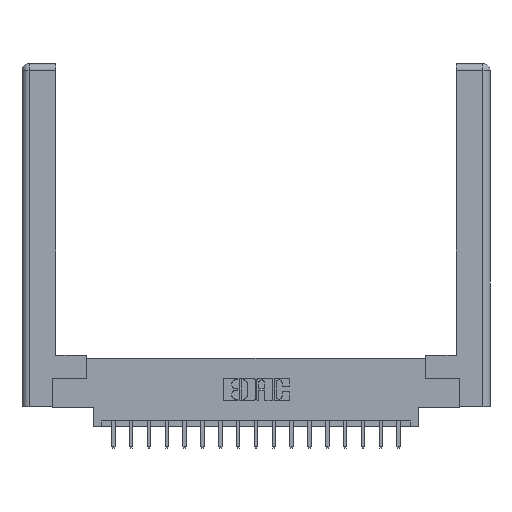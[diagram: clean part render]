
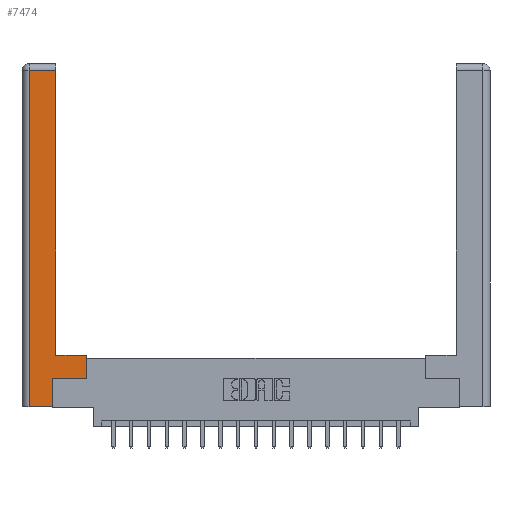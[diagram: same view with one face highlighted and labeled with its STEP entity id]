
A CAD part, top view. The second image highlights one B-rep face of the part: STEP entity #7474.
In plain terms, the highlighted planar face has unit normal (0, 0, 1).
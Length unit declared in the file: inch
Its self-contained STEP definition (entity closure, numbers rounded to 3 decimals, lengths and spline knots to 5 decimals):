
#240 = CARTESIAN_POINT ( 'NONE',  ( 0.295, 3., 0. ) ) ;
#743 = CARTESIAN_POINT ( 'NONE',  ( 0.295, 0.45, 0. ) ) ;
#848 = ORIENTED_EDGE ( 'NONE', *, *, #8095, .T. ) ;
#1612 = EDGE_LOOP ( 'NONE', ( #6051, #14851, #3664, #1820, #11303, #848, #16238, #18744 ) ) ;
#1820 = ORIENTED_EDGE ( 'NONE', *, *, #12712, .T. ) ;
#1840 = CARTESIAN_POINT ( 'NONE',  ( 0.565, 0.45, 0. ) ) ;
#2045 = EDGE_CURVE ( 'NONE', #13140, #7228, #2820, .T. ) ;
#2797 = VECTOR ( 'NONE', #11069, 39.37008 ) ;
#2820 = LINE ( 'NONE', #240, #8913 ) ;
#3087 = VERTEX_POINT ( 'NONE', #5712 ) ;
#3099 = AXIS2_PLACEMENT_3D ( 'NONE', #17085, #12384, #15464 ) ;
#3273 = LINE ( 'NONE', #4502, #3928 ) ;
#3664 = ORIENTED_EDGE ( 'NONE', *, *, #7607, .T. ) ;
#3837 = PLANE ( 'NONE',  #3099 ) ;
#3928 = VECTOR ( 'NONE', #10180, 39.37008 ) ;
#4420 = FACE_OUTER_BOUND ( 'NONE', #1612, .T. ) ;
#4452 = CARTESIAN_POINT ( 'NONE',  ( 0.0615, 2.94, 0. ) ) ;
#4502 = CARTESIAN_POINT ( 'NONE',  ( 0.265, 0.245, 0. ) ) ;
#4542 = CARTESIAN_POINT ( 'NONE',  ( 0.565, 0.245, 0. ) ) ;
#5068 = CARTESIAN_POINT ( 'NONE',  ( 0.295, 0.45, 0. ) ) ;
#5265 = VECTOR ( 'NONE', #14887, 39.37008 ) ;
#5712 = CARTESIAN_POINT ( 'NONE',  ( 0.265, 0., 0. ) ) ;
#6051 = ORIENTED_EDGE ( 'NONE', *, *, #2045, .T. ) ;
#6334 = DIRECTION ( 'NONE',  ( 0., 1., 0. ) ) ;
#6375 = LINE ( 'NONE', #1840, #14058 ) ;
#7228 = VERTEX_POINT ( 'NONE', #14047 ) ;
#7271 = VERTEX_POINT ( 'NONE', #15995 ) ;
#7474 = ADVANCED_FACE ( 'NONE', ( #4420 ), #3837, .F. ) ;
#7607 = EDGE_CURVE ( 'NONE', #18257, #17679, #17495, .T. ) ;
#7945 = DIRECTION ( 'NONE',  ( 0., 1., 0. ) ) ;
#8095 = EDGE_CURVE ( 'NONE', #7271, #8157, #14206, .T. ) ;
#8157 = VERTEX_POINT ( 'NONE', #4542 ) ;
#8913 = VECTOR ( 'NONE', #6334, 39.37008 ) ;
#9352 = LINE ( 'NONE', #743, #2797 ) ;
#9545 = DIRECTION ( 'NONE',  ( 0., -1., 0. ) ) ;
#9573 = VECTOR ( 'NONE', #9545, 39.37008 ) ;
#9794 = EDGE_CURVE ( 'NONE', #17604, #13140, #9352, .T. ) ;
#10180 = DIRECTION ( 'NONE',  ( 0., 1., 0. ) ) ;
#10429 = EDGE_CURVE ( 'NONE', #3087, #7271, #3273, .T. ) ;
#11069 = DIRECTION ( 'NONE',  ( -1., 0., 0. ) ) ;
#11303 = ORIENTED_EDGE ( 'NONE', *, *, #10429, .T. ) ;
#11360 = CARTESIAN_POINT ( 'NONE',  ( 0.565, 0.45, 0. ) ) ;
#11549 = LINE ( 'NONE', #4452, #5265 ) ;
#12154 = EDGE_CURVE ( 'NONE', #7228, #18257, #11549, .T. ) ;
#12261 = VECTOR ( 'NONE', #18531, 39.37008 ) ;
#12326 = VECTOR ( 'NONE', #19212, 39.37008 ) ;
#12384 = DIRECTION ( 'NONE',  ( 0., 0., -1. ) ) ;
#12712 = EDGE_CURVE ( 'NONE', #17679, #3087, #17409, .T. ) ;
#13140 = VERTEX_POINT ( 'NONE', #5068 ) ;
#14047 = CARTESIAN_POINT ( 'NONE',  ( 0.295, 2.94, 0. ) ) ;
#14058 = VECTOR ( 'NONE', #7945, 39.37008 ) ;
#14081 = CARTESIAN_POINT ( 'NONE',  ( 0.265, 0., 0. ) ) ;
#14206 = LINE ( 'NONE', #14645, #12326 ) ;
#14210 = CARTESIAN_POINT ( 'NONE',  ( 0.0615, 0., 0. ) ) ;
#14645 = CARTESIAN_POINT ( 'NONE',  ( 0.565, 0.245, 0. ) ) ;
#14851 = ORIENTED_EDGE ( 'NONE', *, *, #12154, .T. ) ;
#14887 = DIRECTION ( 'NONE',  ( -1., 0., 0. ) ) ;
#15464 = DIRECTION ( 'NONE',  ( -1., 0., 0. ) ) ;
#15995 = CARTESIAN_POINT ( 'NONE',  ( 0.265, 0.245, 0. ) ) ;
#16238 = ORIENTED_EDGE ( 'NONE', *, *, #16398, .T. ) ;
#16316 = CARTESIAN_POINT ( 'NONE',  ( 0.0615, 0., 0. ) ) ;
#16398 = EDGE_CURVE ( 'NONE', #8157, #17604, #6375, .T. ) ;
#17085 = CARTESIAN_POINT ( 'NONE',  ( 0., 0., 0. ) ) ;
#17409 = LINE ( 'NONE', #14081, #12261 ) ;
#17495 = LINE ( 'NONE', #14210, #9573 ) ;
#17604 = VERTEX_POINT ( 'NONE', #11360 ) ;
#17679 = VERTEX_POINT ( 'NONE', #16316 ) ;
#18257 = VERTEX_POINT ( 'NONE', #19136 ) ;
#18531 = DIRECTION ( 'NONE',  ( 1., 0., 0. ) ) ;
#18744 = ORIENTED_EDGE ( 'NONE', *, *, #9794, .T. ) ;
#19136 = CARTESIAN_POINT ( 'NONE',  ( 0.0615, 2.94, 0. ) ) ;
#19212 = DIRECTION ( 'NONE',  ( 1., 0., 0. ) ) ;
